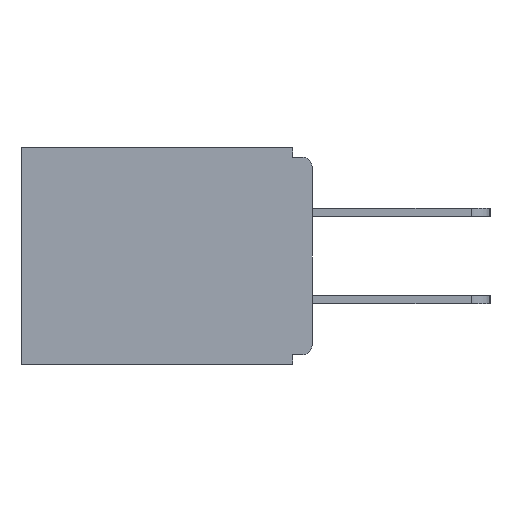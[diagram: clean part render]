
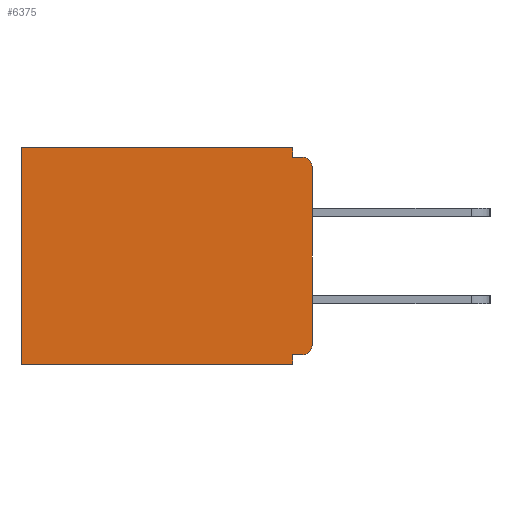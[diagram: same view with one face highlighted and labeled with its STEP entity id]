
A CAD part, left-side view. The second image highlights one B-rep face of the part: STEP entity #6375.
In plain terms, the highlighted planar face has unit normal (-1, 0, 0).
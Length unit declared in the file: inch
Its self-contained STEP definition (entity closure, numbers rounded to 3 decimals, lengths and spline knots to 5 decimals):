
#121 = VERTEX_POINT ( 'NONE', #2533 ) ;
#194 = DIRECTION ( 'NONE',  ( 0., 0., -1. ) ) ;
#384 = LINE ( 'NONE', #6471, #13456 ) ;
#788 = LINE ( 'NONE', #6005, #2544 ) ;
#948 = LINE ( 'NONE', #10611, #2903 ) ;
#982 = DIRECTION ( 'NONE',  ( -1., 0., 0. ) ) ;
#1042 = VERTEX_POINT ( 'NONE', #12088 ) ;
#1096 = EDGE_CURVE ( 'NONE', #10372, #8404, #6487, .T. ) ;
#1411 = LINE ( 'NONE', #12252, #4991 ) ;
#1621 = ORIENTED_EDGE ( 'NONE', *, *, #8126, .F. ) ;
#2221 = DIRECTION ( 'NONE',  ( 0., 1., 0. ) ) ;
#2533 = CARTESIAN_POINT ( 'NONE',  ( 0.298, 0.015, -0.015 ) ) ;
#2544 = VECTOR ( 'NONE', #15129, 39.37008 ) ;
#2728 = CARTESIAN_POINT ( 'NONE',  ( 0.298, 0., -0.313 ) ) ;
#2903 = VECTOR ( 'NONE', #9157, 39.37008 ) ;
#3419 = EDGE_CURVE ( 'NONE', #11328, #3624, #14739, .T. ) ;
#3616 = VECTOR ( 'NONE', #194, 39.37008 ) ;
#3624 = VERTEX_POINT ( 'NONE', #11530 ) ;
#3644 = DIRECTION ( 'NONE',  ( 0., 1., 0. ) ) ;
#3688 = CARTESIAN_POINT ( 'NONE',  ( 0.298, 0.031, 0. ) ) ;
#4255 = CARTESIAN_POINT ( 'NONE',  ( 0.298, 0., -0.328 ) ) ;
#4374 = ORIENTED_EDGE ( 'NONE', *, *, #9406, .F. ) ;
#4656 = EDGE_CURVE ( 'NONE', #3624, #5161, #14118, .T. ) ;
#4710 = CARTESIAN_POINT ( 'NONE',  ( 0.298, 0.015, -0.328 ) ) ;
#4991 = VECTOR ( 'NONE', #3644, 39.37008 ) ;
#5028 = EDGE_CURVE ( 'NONE', #10372, #7007, #12340, .T. ) ;
#5161 = VERTEX_POINT ( 'NONE', #7146 ) ;
#5212 = PLANE ( 'NONE',  #13391 ) ;
#5259 = EDGE_CURVE ( 'NONE', #1042, #121, #10770, .T. ) ;
#5723 = VERTEX_POINT ( 'NONE', #7337 ) ;
#5751 = CARTESIAN_POINT ( 'NONE',  ( 0.298, 0.015, -0.313 ) ) ;
#5805 = DIRECTION ( 'NONE',  ( 0., -1., 0. ) ) ;
#5852 = ORIENTED_EDGE ( 'NONE', *, *, #5028, .T. ) ;
#6005 = CARTESIAN_POINT ( 'NONE',  ( 0.298, 0.031, -0.343 ) ) ;
#6347 = CARTESIAN_POINT ( 'NONE',  ( 0.298, 0., 0. ) ) ;
#6375 = ADVANCED_FACE ( 'NONE', ( #6405 ), #5212, .F. ) ;
#6405 = FACE_OUTER_BOUND ( 'NONE', #9496, .T. ) ;
#6469 = VERTEX_POINT ( 'NONE', #11743 ) ;
#6471 = CARTESIAN_POINT ( 'NONE',  ( 0.298, 0., 0. ) ) ;
#6487 = LINE ( 'NONE', #4255, #10897 ) ;
#6972 = VECTOR ( 'NONE', #5805, 39.37008 ) ;
#7007 = VERTEX_POINT ( 'NONE', #2728 ) ;
#7014 = DIRECTION ( 'NONE',  ( 0., 0., -1. ) ) ;
#7065 = CARTESIAN_POINT ( 'NONE',  ( 0.298, 0.031, -0.328 ) ) ;
#7146 = CARTESIAN_POINT ( 'NONE',  ( 0.298, 0.46, -0.343 ) ) ;
#7289 = CARTESIAN_POINT ( 'NONE',  ( 0.298, 0.015, -0.03 ) ) ;
#7337 = CARTESIAN_POINT ( 'NONE',  ( 0.298, 0., -0.03 ) ) ;
#7395 = CARTESIAN_POINT ( 'NONE',  ( 0.298, 0., 0. ) ) ;
#7485 = ORIENTED_EDGE ( 'NONE', *, *, #1096, .F. ) ;
#8094 = DIRECTION ( 'NONE',  ( 0., 1., 0. ) ) ;
#8126 = EDGE_CURVE ( 'NONE', #6469, #5161, #1411, .T. ) ;
#8404 = VERTEX_POINT ( 'NONE', #7065 ) ;
#8547 = ORIENTED_EDGE ( 'NONE', *, *, #5259, .F. ) ;
#9157 = DIRECTION ( 'NONE',  ( 0., 0., -1. ) ) ;
#9247 = EDGE_CURVE ( 'NONE', #5723, #7007, #384, .T. ) ;
#9390 = ORIENTED_EDGE ( 'NONE', *, *, #3419, .T. ) ;
#9406 = EDGE_CURVE ( 'NONE', #11328, #1042, #788, .T. ) ;
#9496 = EDGE_LOOP ( 'NONE', ( #11989, #8547, #4374, #9390, #11977, #1621, #15935, #7485, #5852, #14157 ) ) ;
#10372 = VERTEX_POINT ( 'NONE', #4710 ) ;
#10611 = CARTESIAN_POINT ( 'NONE',  ( 0.298, 0.031, -0.343 ) ) ;
#10770 = LINE ( 'NONE', #15472, #6972 ) ;
#10897 = VECTOR ( 'NONE', #8094, 39.37008 ) ;
#11328 = VERTEX_POINT ( 'NONE', #3688 ) ;
#11479 = CARTESIAN_POINT ( 'NONE',  ( 0.298, 0.46, 0. ) ) ;
#11530 = CARTESIAN_POINT ( 'NONE',  ( 0.298, 0.46, 0. ) ) ;
#11743 = CARTESIAN_POINT ( 'NONE',  ( 0.298, 0.031, -0.343 ) ) ;
#11820 = AXIS2_PLACEMENT_3D ( 'NONE', #5751, #14604, #7014 ) ;
#11937 = EDGE_CURVE ( 'NONE', #8404, #6469, #948, .T. ) ;
#11977 = ORIENTED_EDGE ( 'NONE', *, *, #4656, .T. ) ;
#11989 = ORIENTED_EDGE ( 'NONE', *, *, #13380, .T. ) ;
#12088 = CARTESIAN_POINT ( 'NONE',  ( 0.298, 0.031, -0.015 ) ) ;
#12220 = CIRCLE ( 'NONE', #14234, 0.015 ) ;
#12252 = CARTESIAN_POINT ( 'NONE',  ( 0.298, 0., -0.343 ) ) ;
#12340 = CIRCLE ( 'NONE', #11820, 0.015 ) ;
#12835 = DIRECTION ( 'NONE',  ( 0., 0., -1. ) ) ;
#13343 = VECTOR ( 'NONE', #2221, 39.37008 ) ;
#13380 = EDGE_CURVE ( 'NONE', #5723, #121, #12220, .T. ) ;
#13391 = AXIS2_PLACEMENT_3D ( 'NONE', #6347, #15315, #12835 ) ;
#13456 = VECTOR ( 'NONE', #14741, 39.37008 ) ;
#13634 = DIRECTION ( 'NONE',  ( 0., 0., -1. ) ) ;
#14118 = LINE ( 'NONE', #11479, #3616 ) ;
#14157 = ORIENTED_EDGE ( 'NONE', *, *, #9247, .F. ) ;
#14234 = AXIS2_PLACEMENT_3D ( 'NONE', #7289, #982, #13634 ) ;
#14604 = DIRECTION ( 'NONE',  ( -1., 0., 0. ) ) ;
#14739 = LINE ( 'NONE', #7395, #13343 ) ;
#14741 = DIRECTION ( 'NONE',  ( 0., 0., -1. ) ) ;
#15129 = DIRECTION ( 'NONE',  ( 0., 0., -1. ) ) ;
#15315 = DIRECTION ( 'NONE',  ( 1., 0., 0. ) ) ;
#15472 = CARTESIAN_POINT ( 'NONE',  ( 0.298, 0., -0.015 ) ) ;
#15935 = ORIENTED_EDGE ( 'NONE', *, *, #11937, .F. ) ;
